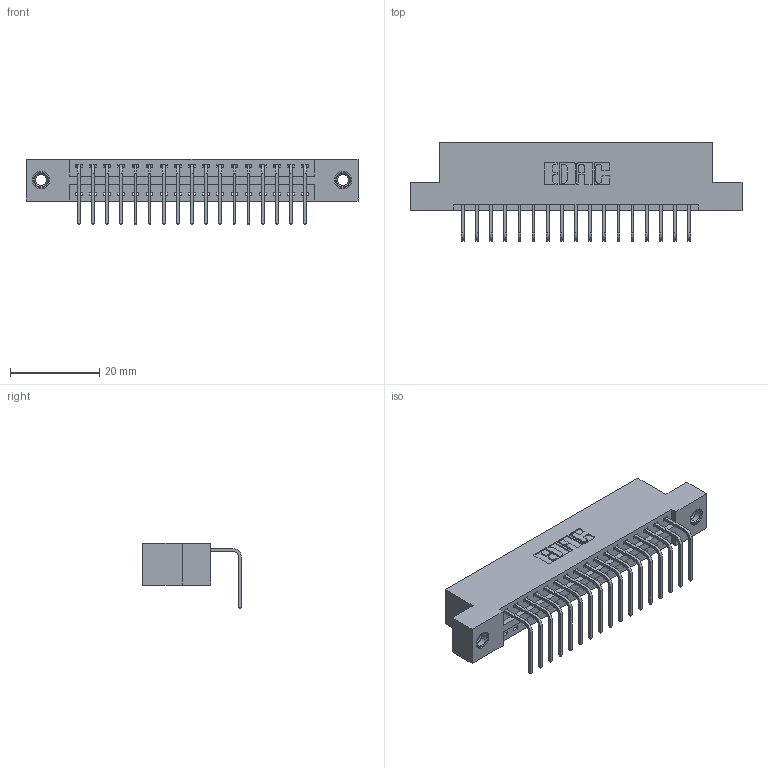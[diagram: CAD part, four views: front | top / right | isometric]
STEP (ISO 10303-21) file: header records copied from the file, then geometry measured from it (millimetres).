
FILE_DESCRIPTION (( 'STEP AP203' ), '1' );
FILE_NAME ('346-017-558-107.STEP', '2022-05-05T13:25:11', ( '' ), ( '' ), 'SwSTEP 2.0', 'SolidWorks 2020', '' );
FILE_SCHEMA (( 'CONFIG_CONTROL_DESIGN' ));
Length unit declared in the file: inch
Products named in the file (4): 346-017-558-107; 345-292-001_558 Tail - 2; 346 Part_Flush Mounting Lugs - 0.156 Dia-TI; 345-250-001_345-250-005-103
Assembly tree (20 placements, depth 2):
  346-017-558-107
    346 Part_Flush Mounting Lugs - 0.156 Dia-TI
    345-292-001_558 Tail - 2  x17
    345-250-001_345-250-005-103  x2
Bounding box: 74.55 x 22.16 x 14.73 mm (x, y, z)
Volume: 7006.9 mm3; surface area: 8860.5 mm2
Topology: 20 solids, 20 shells, 1202 faces, 3559 edges, 2342 vertices
Faces by surface type: plane 822, cylinder 364, cone 12, torus 4
Entity records: 15186 total; most frequent: CARTESIAN_POINT 2594, ORIENTED_EDGE 2538, DIRECTION 2345, EDGE_CURVE 1269, LINE 1049, VECTOR 1049, VERTEX_POINT 840, AXIS2_PLACEMENT_3D 648
